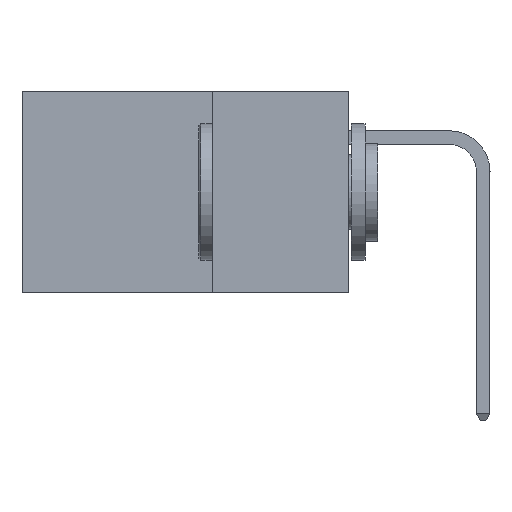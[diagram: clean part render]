
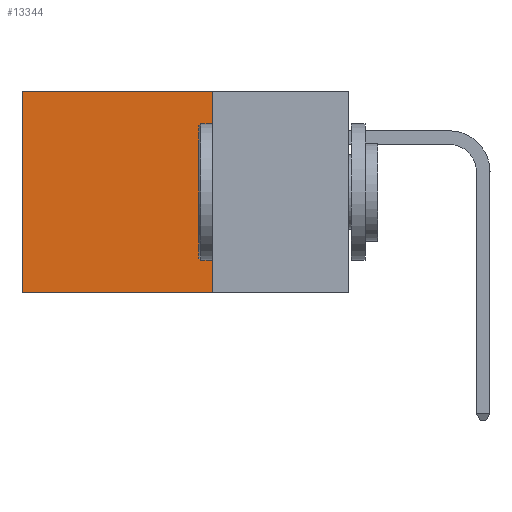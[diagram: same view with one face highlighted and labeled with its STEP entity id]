
A CAD part, left-side view. The second image highlights one B-rep face of the part: STEP entity #13344.
In plain terms, the highlighted planar face has unit normal (-1, 0, 0).
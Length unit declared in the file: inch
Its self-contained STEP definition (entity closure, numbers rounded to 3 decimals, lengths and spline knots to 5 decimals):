
#2145 = EDGE_CURVE ( 'NONE', #11618, #10840, #4338, .T. ) ;
#2379 = DIRECTION ( 'NONE',  ( 0., 0., -1. ) ) ;
#3089 = LINE ( 'NONE', #10420, #13778 ) ;
#3321 = ORIENTED_EDGE ( 'NONE', *, *, #12569, .F. ) ;
#3837 = CARTESIAN_POINT ( 'NONE',  ( 0.2875, 0.6, -0.37 ) ) ;
#4338 = LINE ( 'NONE', #6386, #15394 ) ;
#4611 = ORIENTED_EDGE ( 'NONE', *, *, #7350, .T. ) ;
#5213 = ORIENTED_EDGE ( 'NONE', *, *, #6001, .T. ) ;
#6001 = EDGE_CURVE ( 'NONE', #13143, #10840, #3089, .T. ) ;
#6386 = CARTESIAN_POINT ( 'NONE',  ( 0.2875, 0.25, -0.37 ) ) ;
#6613 = CARTESIAN_POINT ( 'NONE',  ( 0.2875, 0.25, 0. ) ) ;
#6942 = CARTESIAN_POINT ( 'NONE',  ( 0.2875, 0.25, 0. ) ) ;
#6952 = CARTESIAN_POINT ( 'NONE',  ( 0.2875, 0.25, -0.37 ) ) ;
#7350 = EDGE_CURVE ( 'NONE', #10734, #13143, #7661, .T. ) ;
#7661 = LINE ( 'NONE', #7812, #10888 ) ;
#7812 = CARTESIAN_POINT ( 'NONE',  ( 0.2875, 0.25, 0. ) ) ;
#8033 = ORIENTED_EDGE ( 'NONE', *, *, #2145, .F. ) ;
#8335 = DIRECTION ( 'NONE',  ( 0., 0., -1. ) ) ;
#9164 = DIRECTION ( 'NONE',  ( 0., 1., 0. ) ) ;
#9473 = DIRECTION ( 'NONE',  ( 0., 1., 0. ) ) ;
#10420 = CARTESIAN_POINT ( 'NONE',  ( 0.2875, 0.6, 0. ) ) ;
#10591 = CARTESIAN_POINT ( 'NONE',  ( 0.2875, 0.6, 0. ) ) ;
#10734 = VERTEX_POINT ( 'NONE', #17268 ) ;
#10840 = VERTEX_POINT ( 'NONE', #3837 ) ;
#10888 = VECTOR ( 'NONE', #9164, 39.37008 ) ;
#11108 = VECTOR ( 'NONE', #2379, 39.37008 ) ;
#11618 = VERTEX_POINT ( 'NONE', #6952 ) ;
#12448 = PLANE ( 'NONE',  #14523 ) ;
#12569 = EDGE_CURVE ( 'NONE', #10734, #11618, #14369, .T. ) ;
#13143 = VERTEX_POINT ( 'NONE', #10591 ) ;
#13280 = EDGE_LOOP ( 'NONE', ( #5213, #8033, #3321, #4611 ) ) ;
#13344 = ADVANCED_FACE ( 'NONE', ( #17066 ), #12448, .F. ) ;
#13778 = VECTOR ( 'NONE', #17276, 39.37008 ) ;
#14369 = LINE ( 'NONE', #6613, #11108 ) ;
#14523 = AXIS2_PLACEMENT_3D ( 'NONE', #6942, #16515, #8335 ) ;
#15394 = VECTOR ( 'NONE', #9473, 39.37008 ) ;
#16515 = DIRECTION ( 'NONE',  ( 1., 0., 0. ) ) ;
#17066 = FACE_OUTER_BOUND ( 'NONE', #13280, .T. ) ;
#17268 = CARTESIAN_POINT ( 'NONE',  ( 0.2875, 0.25, 0. ) ) ;
#17276 = DIRECTION ( 'NONE',  ( 0., 0., -1. ) ) ;
